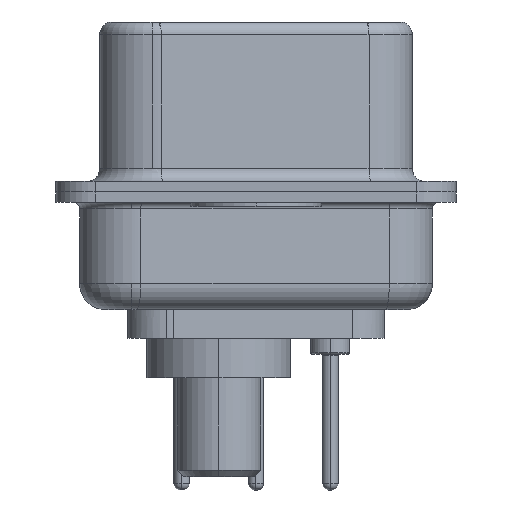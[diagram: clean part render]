
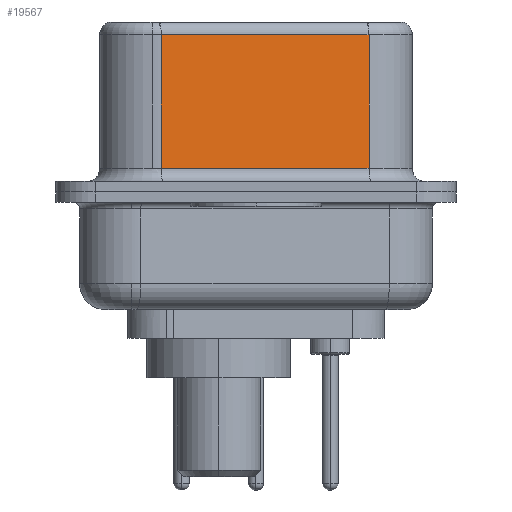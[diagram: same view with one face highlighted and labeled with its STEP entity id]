
A CAD part, left-side view. The second image highlights one B-rep face of the part: STEP entity #19567.
In plain terms, the highlighted planar face has unit normal (-0.985, -0.174, 0).
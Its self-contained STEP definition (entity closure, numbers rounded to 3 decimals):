
#534 = CARTESIAN_POINT ( 'NONE',  ( 5.132, -4.322, 6.02 ) ) ;
#711 = ORIENTED_EDGE ( 'NONE', *, *, #7703, .T. ) ;
#2493 = EDGE_CURVE ( 'NONE', #21715, #21256, #5507, .T. ) ;
#2499 = AXIS2_PLACEMENT_3D ( 'NONE', #3342, #16580, #5284 ) ;
#3342 = CARTESIAN_POINT ( 'NONE',  ( 5.132, -4.322, 6.52 ) ) ;
#3788 = CARTESIAN_POINT ( 'NONE',  ( 5.132, -4.322, 0.9 ) ) ;
#4765 = EDGE_CURVE ( 'NONE', #21715, #23460, #7907, .T. ) ;
#5103 = CARTESIAN_POINT ( 'NONE',  ( 3.73, 3.628, 6.52 ) ) ;
#5215 = ORIENTED_EDGE ( 'NONE', *, *, #22572, .T. ) ;
#5284 = DIRECTION ( 'NONE',  ( -0.174, 0.985, 0. ) ) ;
#5507 = LINE ( 'NONE', #19434, #19906 ) ;
#7703 = EDGE_CURVE ( 'NONE', #11700, #21256, #20007, .T. ) ;
#7907 = LINE ( 'NONE', #21252, #22806 ) ;
#9736 = ORIENTED_EDGE ( 'NONE', *, *, #2493, .F. ) ;
#9777 = CARTESIAN_POINT ( 'NONE',  ( 3.73, 3.628, 6.02 ) ) ;
#11700 = VERTEX_POINT ( 'NONE', #16696 ) ;
#13344 = DIRECTION ( 'NONE',  ( 0.174, -0.985, 0. ) ) ;
#14686 = ORIENTED_EDGE ( 'NONE', *, *, #4765, .T. ) ;
#14710 = PLANE ( 'NONE',  #2499 ) ;
#16412 = DIRECTION ( 'NONE',  ( 0., 0., -1. ) ) ;
#16580 = DIRECTION ( 'NONE',  ( 0.985, 0.174, 0. ) ) ;
#16696 = CARTESIAN_POINT ( 'NONE',  ( 3.73, 3.628, 0.9 ) ) ;
#17730 = DIRECTION ( 'NONE',  ( -0.174, 0.985, 0. ) ) ;
#17961 = CARTESIAN_POINT ( 'NONE',  ( 5.132, -4.322, 0.9 ) ) ;
#19062 = DIRECTION ( 'NONE',  ( 0., 0., -1. ) ) ;
#19434 = CARTESIAN_POINT ( 'NONE',  ( 5.132, -4.322, 6.52 ) ) ;
#19567 = ADVANCED_FACE ( 'NONE', ( #20299 ), #14710, .F. ) ;
#19906 = VECTOR ( 'NONE', #19062, 1000. ) ;
#20007 = LINE ( 'NONE', #3788, #24417 ) ;
#20299 = FACE_OUTER_BOUND ( 'NONE', #22685, .T. ) ;
#21252 = CARTESIAN_POINT ( 'NONE',  ( 5.132, -4.322, 6.02 ) ) ;
#21256 = VERTEX_POINT ( 'NONE', #17961 ) ;
#21651 = VECTOR ( 'NONE', #16412, 1000. ) ;
#21715 = VERTEX_POINT ( 'NONE', #534 ) ;
#22226 = LINE ( 'NONE', #5103, #21651 ) ;
#22572 = EDGE_CURVE ( 'NONE', #23460, #11700, #22226, .T. ) ;
#22685 = EDGE_LOOP ( 'NONE', ( #9736, #14686, #5215, #711 ) ) ;
#22806 = VECTOR ( 'NONE', #17730, 1000. ) ;
#23460 = VERTEX_POINT ( 'NONE', #9777 ) ;
#24417 = VECTOR ( 'NONE', #13344, 1000. ) ;
